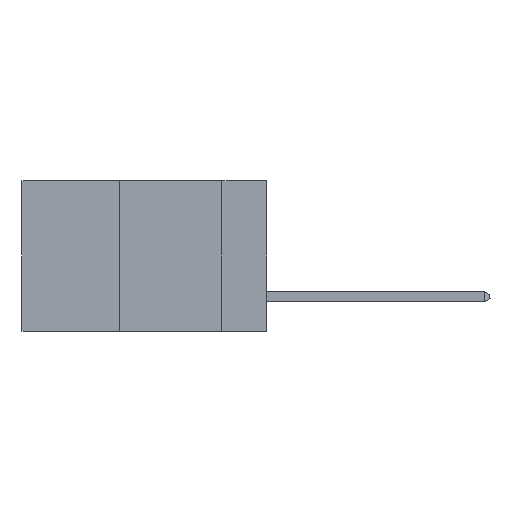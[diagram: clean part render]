
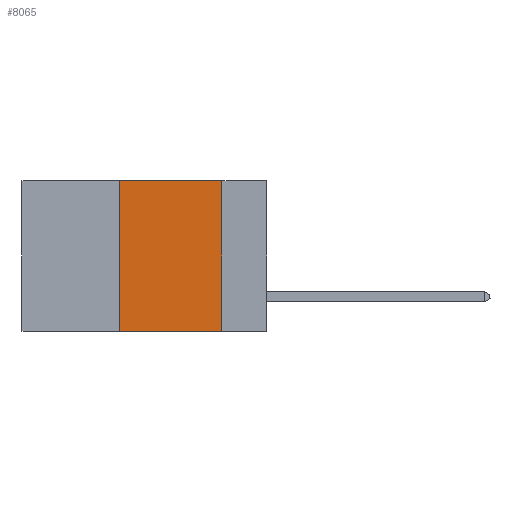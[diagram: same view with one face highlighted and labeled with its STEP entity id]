
A CAD part, left-side view. The second image highlights one B-rep face of the part: STEP entity #8065.
In plain terms, the highlighted planar face has unit normal (-1, 0, 0).
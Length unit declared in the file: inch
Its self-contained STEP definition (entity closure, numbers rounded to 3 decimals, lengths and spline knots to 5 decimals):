
#251 = CARTESIAN_POINT ( 'NONE',  ( 0., 0.6, -0.37 ) ) ;
#415 = ORIENTED_EDGE ( 'NONE', *, *, #4995, .F. ) ;
#487 = VECTOR ( 'NONE', #9270, 39.37008 ) ;
#966 = DIRECTION ( 'NONE',  ( 0., 0., -1. ) ) ;
#1105 = LINE ( 'NONE', #251, #11040 ) ;
#1273 = ORIENTED_EDGE ( 'NONE', *, *, #10256, .T. ) ;
#2065 = DIRECTION ( 'NONE',  ( 0., -1., 0. ) ) ;
#2198 = DIRECTION ( 'NONE',  ( 0., -1., 0. ) ) ;
#2251 = VERTEX_POINT ( 'NONE', #3170 ) ;
#3082 = CARTESIAN_POINT ( 'NONE',  ( 0., 0.11, 0. ) ) ;
#3170 = CARTESIAN_POINT ( 'NONE',  ( 0., 0.36, -0.37 ) ) ;
#3414 = LINE ( 'NONE', #3082, #11756 ) ;
#3540 = LINE ( 'NONE', #5475, #487 ) ;
#4995 = EDGE_CURVE ( 'NONE', #9523, #7445, #8308, .T. ) ;
#5467 = CARTESIAN_POINT ( 'NONE',  ( 0., 0.36, 0. ) ) ;
#5475 = CARTESIAN_POINT ( 'NONE',  ( 0., 0.36, 0. ) ) ;
#5537 = DIRECTION ( 'NONE',  ( 1., 0., 0. ) ) ;
#5880 = CARTESIAN_POINT ( 'NONE',  ( 0., 0.6, 0. ) ) ;
#6434 = CARTESIAN_POINT ( 'NONE',  ( 0., 0.6, 0. ) ) ;
#6654 = VERTEX_POINT ( 'NONE', #7698 ) ;
#7445 = VERTEX_POINT ( 'NONE', #8781 ) ;
#7479 = ORIENTED_EDGE ( 'NONE', *, *, #10323, .F. ) ;
#7698 = CARTESIAN_POINT ( 'NONE',  ( 0., 0.11, -0.37 ) ) ;
#8007 = VECTOR ( 'NONE', #2065, 39.37008 ) ;
#8041 = ORIENTED_EDGE ( 'NONE', *, *, #11594, .F. ) ;
#8065 = ADVANCED_FACE ( 'NONE', ( #11356 ), #10049, .F. ) ;
#8308 = LINE ( 'NONE', #5880, #8007 ) ;
#8436 = AXIS2_PLACEMENT_3D ( 'NONE', #6434, #5537, #966 ) ;
#8781 = CARTESIAN_POINT ( 'NONE',  ( 0., 0.11, 0. ) ) ;
#9270 = DIRECTION ( 'NONE',  ( 0., 0., 1. ) ) ;
#9523 = VERTEX_POINT ( 'NONE', #5467 ) ;
#10049 = PLANE ( 'NONE',  #8436 ) ;
#10256 = EDGE_CURVE ( 'NONE', #2251, #6654, #1105, .T. ) ;
#10323 = EDGE_CURVE ( 'NONE', #7445, #6654, #3414, .T. ) ;
#10605 = DIRECTION ( 'NONE',  ( 0., 0., -1. ) ) ;
#11040 = VECTOR ( 'NONE', #2198, 39.37008 ) ;
#11356 = FACE_OUTER_BOUND ( 'NONE', #11636, .T. ) ;
#11594 = EDGE_CURVE ( 'NONE', #2251, #9523, #3540, .T. ) ;
#11636 = EDGE_LOOP ( 'NONE', ( #7479, #415, #8041, #1273 ) ) ;
#11756 = VECTOR ( 'NONE', #10605, 39.37008 ) ;
